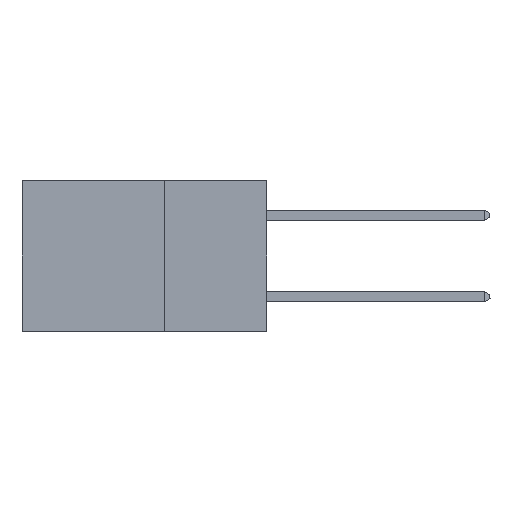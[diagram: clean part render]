
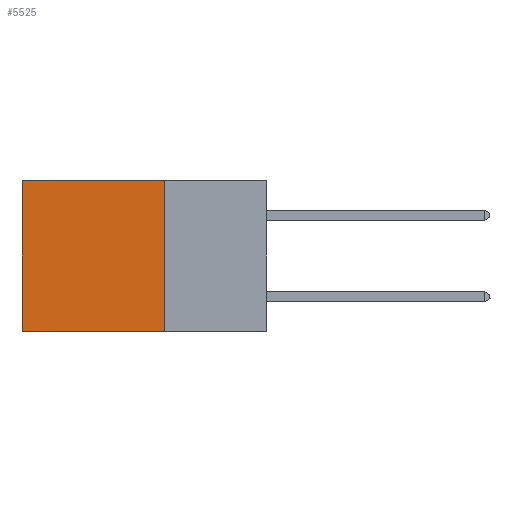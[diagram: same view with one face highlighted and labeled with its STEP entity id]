
A CAD part, left-side view. The second image highlights one B-rep face of the part: STEP entity #5525.
In plain terms, the highlighted planar face has unit normal (-1, 0, 0).
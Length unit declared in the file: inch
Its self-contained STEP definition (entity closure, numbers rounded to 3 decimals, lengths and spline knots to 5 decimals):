
#1264 = DIRECTION ( 'NONE',  ( 0., 1., 0. ) ) ;
#1574 = EDGE_LOOP ( 'NONE', ( #16868, #10268, #4946, #10112 ) ) ;
#3224 = CARTESIAN_POINT ( 'NONE',  ( 0.2875, 0.25, 0. ) ) ;
#3393 = EDGE_CURVE ( 'NONE', #18577, #11020, #18632, .T. ) ;
#3756 = LINE ( 'NONE', #3224, #7411 ) ;
#4064 = VERTEX_POINT ( 'NONE', #11115 ) ;
#4352 = AXIS2_PLACEMENT_3D ( 'NONE', #16301, #19831, #13037 ) ;
#4946 = ORIENTED_EDGE ( 'NONE', *, *, #12810, .F. ) ;
#5470 = LINE ( 'NONE', #14756, #18056 ) ;
#5525 = ADVANCED_FACE ( 'NONE', ( #16971 ), #9969, .F. ) ;
#7411 = VECTOR ( 'NONE', #14648, 39.37008 ) ;
#9969 = PLANE ( 'NONE',  #4352 ) ;
#10112 = ORIENTED_EDGE ( 'NONE', *, *, #3393, .T. ) ;
#10268 = ORIENTED_EDGE ( 'NONE', *, *, #17919, .F. ) ;
#10468 = VECTOR ( 'NONE', #1264, 39.37008 ) ;
#11020 = VERTEX_POINT ( 'NONE', #14731 ) ;
#11115 = CARTESIAN_POINT ( 'NONE',  ( 0.2875, 0.25, -0.37 ) ) ;
#11143 = LINE ( 'NONE', #14732, #12133 ) ;
#11609 = CARTESIAN_POINT ( 'NONE',  ( 0.2875, 0.6, -0.37 ) ) ;
#12133 = VECTOR ( 'NONE', #14795, 39.37008 ) ;
#12281 = VERTEX_POINT ( 'NONE', #11609 ) ;
#12810 = EDGE_CURVE ( 'NONE', #18577, #4064, #3756, .T. ) ;
#13037 = DIRECTION ( 'NONE',  ( 0., 0., -1. ) ) ;
#14648 = DIRECTION ( 'NONE',  ( 0., 0., -1. ) ) ;
#14731 = CARTESIAN_POINT ( 'NONE',  ( 0.2875, 0.6, 0. ) ) ;
#14732 = CARTESIAN_POINT ( 'NONE',  ( 0.2875, 0.25, -0.37 ) ) ;
#14756 = CARTESIAN_POINT ( 'NONE',  ( 0.2875, 0.6, 0. ) ) ;
#14795 = DIRECTION ( 'NONE',  ( 0., 1., 0. ) ) ;
#15166 = EDGE_CURVE ( 'NONE', #11020, #12281, #5470, .T. ) ;
#15692 = CARTESIAN_POINT ( 'NONE',  ( 0.2875, 0.25, 0. ) ) ;
#16301 = CARTESIAN_POINT ( 'NONE',  ( 0.2875, 0.25, 0. ) ) ;
#16813 = CARTESIAN_POINT ( 'NONE',  ( 0.2875, 0.25, 0. ) ) ;
#16868 = ORIENTED_EDGE ( 'NONE', *, *, #15166, .T. ) ;
#16971 = FACE_OUTER_BOUND ( 'NONE', #1574, .T. ) ;
#17919 = EDGE_CURVE ( 'NONE', #4064, #12281, #11143, .T. ) ;
#18056 = VECTOR ( 'NONE', #18081, 39.37008 ) ;
#18081 = DIRECTION ( 'NONE',  ( 0., 0., -1. ) ) ;
#18577 = VERTEX_POINT ( 'NONE', #16813 ) ;
#18632 = LINE ( 'NONE', #15692, #10468 ) ;
#19831 = DIRECTION ( 'NONE',  ( 1., 0., 0. ) ) ;
